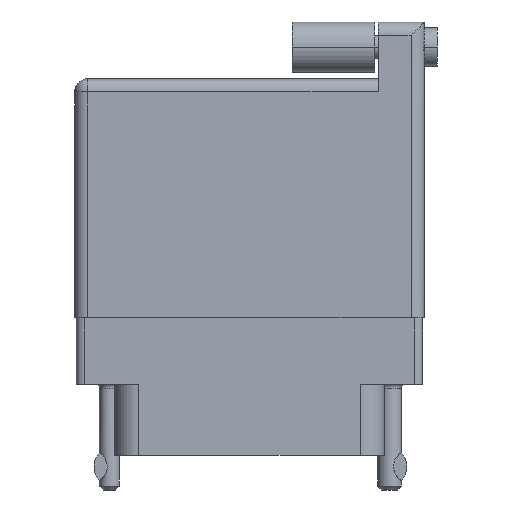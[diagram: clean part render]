
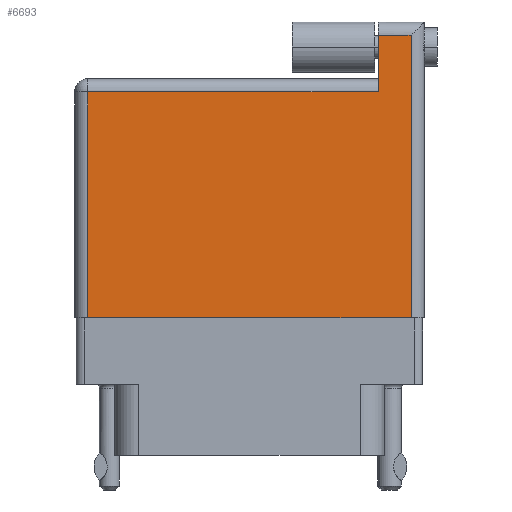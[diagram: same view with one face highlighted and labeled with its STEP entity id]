
A CAD part, front view. The second image highlights one B-rep face of the part: STEP entity #6693.
In plain terms, the highlighted face is planar.
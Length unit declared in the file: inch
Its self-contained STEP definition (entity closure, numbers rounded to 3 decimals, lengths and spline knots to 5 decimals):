
#3528 = CARTESIAN_POINT ( 'NONE',  ( 1.275, 1.07, 0. ) ) ;
#3657 = CARTESIAN_POINT ( 'NONE',  ( 1.275, 1.12, 0. ) ) ;
#6656 = VERTEX_POINT ( 'NONE', #27509 ) ;
#6693 = ADVANCED_FACE ( 'NONE', ( #22601 ), #8831, .F. ) ;
#6822 = CARTESIAN_POINT ( 'NONE',  ( 1.15, 1.12, 0. ) ) ;
#7013 = LINE ( 'NONE', #6822, #25926 ) ;
#7105 = CARTESIAN_POINT ( 'NONE',  ( 1.275, 0., 0. ) ) ;
#7979 = VECTOR ( 'NONE', #14533, 39.37008 ) ;
#8831 = PLANE ( 'NONE',  #31691 ) ;
#9418 = VECTOR ( 'NONE', #20363, 39.37008 ) ;
#10044 = DIRECTION ( 'NONE',  ( 1., 0., 0. ) ) ;
#10445 = CARTESIAN_POINT ( 'NONE',  ( 1.15, 1.07, 0. ) ) ;
#10678 = ORIENTED_EDGE ( 'NONE', *, *, #21788, .T. ) ;
#11192 = CARTESIAN_POINT ( 'NONE',  ( 0., 0.906, 0. ) ) ;
#11835 = EDGE_LOOP ( 'NONE', ( #14811, #10678, #20706, #29300, #35207, #32452 ) ) ;
#12396 = LINE ( 'NONE', #28877, #9418 ) ;
#14122 = DIRECTION ( 'NONE',  ( -1., 0., 0. ) ) ;
#14533 = DIRECTION ( 'NONE',  ( 0., 1., 0. ) ) ;
#14811 = ORIENTED_EDGE ( 'NONE', *, *, #32438, .T. ) ;
#17344 = VERTEX_POINT ( 'NONE', #21603 ) ;
#19368 = CARTESIAN_POINT ( 'NONE',  ( 0., 0.856, 0. ) ) ;
#20363 = DIRECTION ( 'NONE',  ( 0., -1., 0. ) ) ;
#20416 = DIRECTION ( 'NONE',  ( 0., -1., 0. ) ) ;
#20531 = LINE ( 'NONE', #20715, #26205 ) ;
#20706 = ORIENTED_EDGE ( 'NONE', *, *, #29877, .T. ) ;
#20715 = CARTESIAN_POINT ( 'NONE',  ( 0., 1.07, 0. ) ) ;
#21272 = LINE ( 'NONE', #31578, #29539 ) ;
#21301 = VERTEX_POINT ( 'NONE', #3528 ) ;
#21603 = CARTESIAN_POINT ( 'NONE',  ( 0.05, 0.856, 0. ) ) ;
#21788 = EDGE_CURVE ( 'NONE', #24184, #21301, #28482, .T. ) ;
#22156 = EDGE_CURVE ( 'NONE', #6656, #17344, #26037, .T. ) ;
#22601 = FACE_OUTER_BOUND ( 'NONE', #11835, .T. ) ;
#23074 = DIRECTION ( 'NONE',  ( -1., 0., 0. ) ) ;
#24184 = VERTEX_POINT ( 'NONE', #7105 ) ;
#25926 = VECTOR ( 'NONE', #20416, 39.37008 ) ;
#26037 = LINE ( 'NONE', #19368, #35760 ) ;
#26205 = VECTOR ( 'NONE', #23074, 39.37008 ) ;
#27352 = VERTEX_POINT ( 'NONE', #10445 ) ;
#27509 = CARTESIAN_POINT ( 'NONE',  ( 1.15, 0.856, 0. ) ) ;
#28034 = DIRECTION ( 'NONE',  ( 0., 0., -1. ) ) ;
#28062 = CARTESIAN_POINT ( 'NONE',  ( 0.05, 0., 0. ) ) ;
#28482 = LINE ( 'NONE', #3657, #7979 ) ;
#28582 = DIRECTION ( 'NONE',  ( -1., 0., 0. ) ) ;
#28877 = CARTESIAN_POINT ( 'NONE',  ( 0.05, 0., 0. ) ) ;
#29300 = ORIENTED_EDGE ( 'NONE', *, *, #33718, .T. ) ;
#29539 = VECTOR ( 'NONE', #10044, 39.37008 ) ;
#29860 = EDGE_CURVE ( 'NONE', #17344, #34442, #12396, .T. ) ;
#29877 = EDGE_CURVE ( 'NONE', #21301, #27352, #20531, .T. ) ;
#31578 = CARTESIAN_POINT ( 'NONE',  ( 0., 0., 0. ) ) ;
#31691 = AXIS2_PLACEMENT_3D ( 'NONE', #11192, #28034, #28582 ) ;
#32438 = EDGE_CURVE ( 'NONE', #34442, #24184, #21272, .T. ) ;
#32452 = ORIENTED_EDGE ( 'NONE', *, *, #29860, .T. ) ;
#33718 = EDGE_CURVE ( 'NONE', #27352, #6656, #7013, .T. ) ;
#34442 = VERTEX_POINT ( 'NONE', #28062 ) ;
#35207 = ORIENTED_EDGE ( 'NONE', *, *, #22156, .T. ) ;
#35760 = VECTOR ( 'NONE', #14122, 39.37008 ) ;
